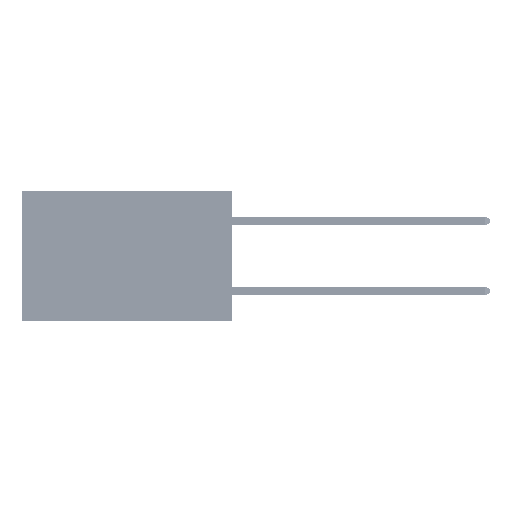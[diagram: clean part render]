
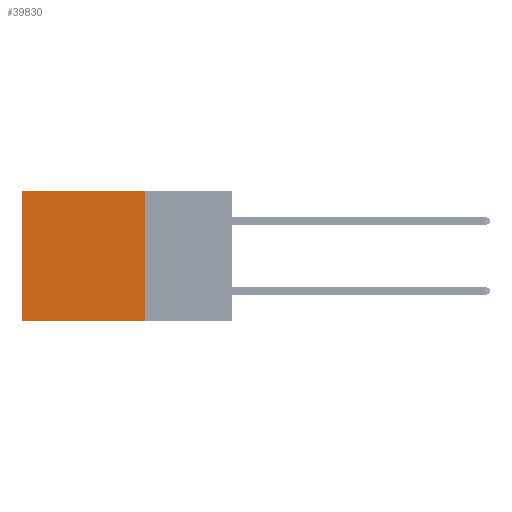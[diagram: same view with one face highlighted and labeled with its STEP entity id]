
A CAD part, left-side view. The second image highlights one B-rep face of the part: STEP entity #39830.
In plain terms, the highlighted planar face has unit normal (-1, 0, 0).
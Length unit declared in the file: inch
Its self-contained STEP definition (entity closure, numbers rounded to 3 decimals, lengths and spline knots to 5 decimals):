
#2064 = CARTESIAN_POINT ( 'NONE',  ( 0.2875, 0.25, -0.37 ) ) ;
#2438 = CARTESIAN_POINT ( 'NONE',  ( 0.2875, 0.6, 0. ) ) ;
#3878 = AXIS2_PLACEMENT_3D ( 'NONE', #48373, #21563, #48540 ) ;
#4191 = CARTESIAN_POINT ( 'NONE',  ( 0.2875, 0.25, 0. ) ) ;
#4712 = VERTEX_POINT ( 'NONE', #2438 ) ;
#5268 = VECTOR ( 'NONE', #32262, 39.37008 ) ;
#5277 = CARTESIAN_POINT ( 'NONE',  ( 0.2875, 0.6, 0. ) ) ;
#6713 = DIRECTION ( 'NONE',  ( 0., 0., -1. ) ) ;
#6754 = EDGE_CURVE ( 'NONE', #36246, #22562, #20720, .T. ) ;
#10056 = CARTESIAN_POINT ( 'NONE',  ( 0.2875, 0.6, -0.37 ) ) ;
#10448 = VERTEX_POINT ( 'NONE', #10056 ) ;
#13084 = LINE ( 'NONE', #5277, #5268 ) ;
#14044 = FACE_OUTER_BOUND ( 'NONE', #16674, .T. ) ;
#15655 = EDGE_CURVE ( 'NONE', #36246, #4712, #45475, .T. ) ;
#15791 = DIRECTION ( 'NONE',  ( 0., 1., 0. ) ) ;
#15872 = VECTOR ( 'NONE', #6713, 39.37008 ) ;
#16674 = EDGE_LOOP ( 'NONE', ( #45605, #27555, #35223, #18076 ) ) ;
#17687 = PLANE ( 'NONE',  #3878 ) ;
#17710 = CARTESIAN_POINT ( 'NONE',  ( 0.2875, 0.25, 0. ) ) ;
#18076 = ORIENTED_EDGE ( 'NONE', *, *, #15655, .T. ) ;
#18416 = DIRECTION ( 'NONE',  ( 0., 1., 0. ) ) ;
#19728 = VECTOR ( 'NONE', #18416, 39.37008 ) ;
#20720 = LINE ( 'NONE', #33386, #15872 ) ;
#21563 = DIRECTION ( 'NONE',  ( 1., 0., 0. ) ) ;
#22562 = VERTEX_POINT ( 'NONE', #2064 ) ;
#23754 = VECTOR ( 'NONE', #15791, 39.37008 ) ;
#27555 = ORIENTED_EDGE ( 'NONE', *, *, #43623, .F. ) ;
#29711 = CARTESIAN_POINT ( 'NONE',  ( 0.2875, 0.25, -0.37 ) ) ;
#32262 = DIRECTION ( 'NONE',  ( 0., 0., -1. ) ) ;
#33085 = EDGE_CURVE ( 'NONE', #4712, #10448, #13084, .T. ) ;
#33386 = CARTESIAN_POINT ( 'NONE',  ( 0.2875, 0.25, 0. ) ) ;
#35223 = ORIENTED_EDGE ( 'NONE', *, *, #6754, .F. ) ;
#36246 = VERTEX_POINT ( 'NONE', #17710 ) ;
#39830 = ADVANCED_FACE ( 'NONE', ( #14044 ), #17687, .F. ) ;
#40275 = LINE ( 'NONE', #29711, #19728 ) ;
#43623 = EDGE_CURVE ( 'NONE', #22562, #10448, #40275, .T. ) ;
#45475 = LINE ( 'NONE', #4191, #23754 ) ;
#45605 = ORIENTED_EDGE ( 'NONE', *, *, #33085, .T. ) ;
#48373 = CARTESIAN_POINT ( 'NONE',  ( 0.2875, 0.25, 0. ) ) ;
#48540 = DIRECTION ( 'NONE',  ( 0., 0., -1. ) ) ;
